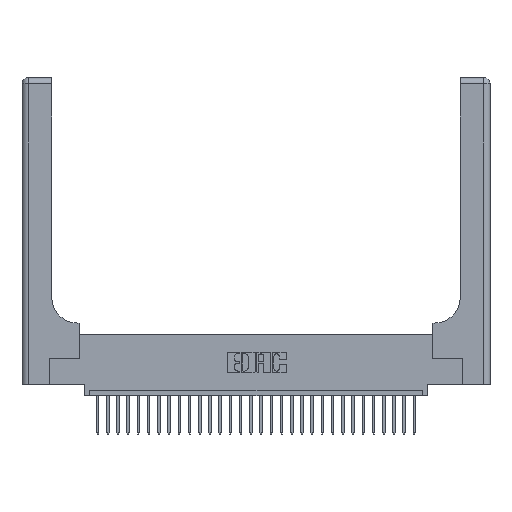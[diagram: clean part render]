
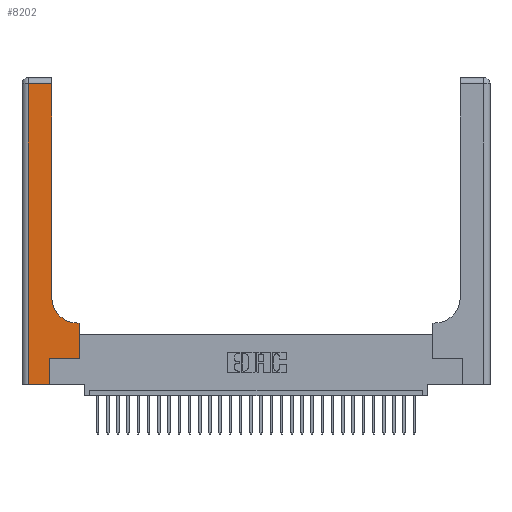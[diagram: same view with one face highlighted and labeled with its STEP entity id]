
A CAD part, top view. The second image highlights one B-rep face of the part: STEP entity #8202.
In plain terms, the highlighted planar face has unit normal (0, 0, 1).
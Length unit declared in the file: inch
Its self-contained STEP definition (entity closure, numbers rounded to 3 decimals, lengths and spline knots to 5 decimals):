
#45 = CARTESIAN_POINT ( 'NONE',  ( 0.06, 0., 0.37 ) ) ;
#70 = CARTESIAN_POINT ( 'NONE',  ( 0.2915, 3., 0.37 ) ) ;
#1363 = LINE ( 'NONE', #4420, #2109 ) ;
#1389 = CARTESIAN_POINT ( 'NONE',  ( 0., 3., 0.37 ) ) ;
#1496 = DIRECTION ( 'NONE',  ( -1., 0., 0. ) ) ;
#1990 = VERTEX_POINT ( 'NONE', #7342 ) ;
#2064 = LINE ( 'NONE', #16189, #18768 ) ;
#2109 = VECTOR ( 'NONE', #21030, 39.37008 ) ;
#2967 = CARTESIAN_POINT ( 'NONE',  ( 0.5415, 0.6, 0.37 ) ) ;
#3401 = CARTESIAN_POINT ( 'NONE',  ( 0.2915, 0.85, 0.37 ) ) ;
#3592 = LINE ( 'NONE', #70, #16576 ) ;
#4128 = DIRECTION ( 'NONE',  ( 0., 1., 0. ) ) ;
#4420 = CARTESIAN_POINT ( 'NONE',  ( 0., 0., 0.37 ) ) ;
#4796 = ORIENTED_EDGE ( 'NONE', *, *, #12431, .T. ) ;
#4954 = VECTOR ( 'NONE', #18918, 39.37008 ) ;
#4992 = ORIENTED_EDGE ( 'NONE', *, *, #6849, .T. ) ;
#5005 = EDGE_CURVE ( 'NONE', #25403, #25594, #29863, .T. ) ;
#5917 = CARTESIAN_POINT ( 'NONE',  ( 0.269, 0.25, 0.37 ) ) ;
#6511 = VERTEX_POINT ( 'NONE', #2967 ) ;
#6522 = EDGE_CURVE ( 'NONE', #28242, #1990, #15727, .T. ) ;
#6849 = EDGE_CURVE ( 'NONE', #29874, #8481, #12381, .T. ) ;
#7317 = CARTESIAN_POINT ( 'NONE',  ( 0.2915, 2.94, 0.37 ) ) ;
#7342 = CARTESIAN_POINT ( 'NONE',  ( 0.5585, 0.6, 0.37 ) ) ;
#8007 = DIRECTION ( 'NONE',  ( 1., 0., 0. ) ) ;
#8202 = ADVANCED_FACE ( 'NONE', ( #24514 ), #29800, .F. ) ;
#8350 = AXIS2_PLACEMENT_3D ( 'NONE', #26307, #9864, #19479 ) ;
#8481 = VERTEX_POINT ( 'NONE', #45 ) ;
#8844 = ORIENTED_EDGE ( 'NONE', *, *, #6522, .T. ) ;
#9443 = CARTESIAN_POINT ( 'NONE',  ( 0.269, 0., 0.37 ) ) ;
#9864 = DIRECTION ( 'NONE',  ( 0., 0., -1. ) ) ;
#10167 = CARTESIAN_POINT ( 'NONE',  ( 0.5585, 0.25, 0.37 ) ) ;
#11515 = CIRCLE ( 'NONE', #8350, 0.25 ) ;
#12280 = EDGE_CURVE ( 'NONE', #25594, #28242, #26995, .T. ) ;
#12381 = LINE ( 'NONE', #25745, #4954 ) ;
#12431 = EDGE_CURVE ( 'NONE', #26972, #29874, #18111, .T. ) ;
#12873 = EDGE_CURVE ( 'NONE', #14348, #26972, #3592, .T. ) ;
#13849 = CARTESIAN_POINT ( 'NONE',  ( 0.269, 0., 0.37 ) ) ;
#14348 = VERTEX_POINT ( 'NONE', #3401 ) ;
#15017 = ORIENTED_EDGE ( 'NONE', *, *, #17464, .T. ) ;
#15727 = LINE ( 'NONE', #10167, #21284 ) ;
#16189 = CARTESIAN_POINT ( 'NONE',  ( 0.2915, 0.6, 0.37 ) ) ;
#16576 = VECTOR ( 'NONE', #4128, 39.37008 ) ;
#17464 = EDGE_CURVE ( 'NONE', #1990, #6511, #2064, .T. ) ;
#18025 = DIRECTION ( 'NONE',  ( 0., 0., -1. ) ) ;
#18111 = LINE ( 'NONE', #29743, #28426 ) ;
#18121 = ORIENTED_EDGE ( 'NONE', *, *, #5005, .T. ) ;
#18755 = CARTESIAN_POINT ( 'NONE',  ( 0.5585, 0.25, 0.37 ) ) ;
#18768 = VECTOR ( 'NONE', #28164, 39.37008 ) ;
#18918 = DIRECTION ( 'NONE',  ( 0., -1., 0. ) ) ;
#19479 = DIRECTION ( 'NONE',  ( 1., 0., 0. ) ) ;
#19800 = ORIENTED_EDGE ( 'NONE', *, *, #28256, .T. ) ;
#20993 = CARTESIAN_POINT ( 'NONE',  ( 0.269, 0.25, 0.37 ) ) ;
#21030 = DIRECTION ( 'NONE',  ( 1., 0., 0. ) ) ;
#21284 = VECTOR ( 'NONE', #24417, 39.37008 ) ;
#21826 = ORIENTED_EDGE ( 'NONE', *, *, #12873, .T. ) ;
#23658 = ORIENTED_EDGE ( 'NONE', *, *, #12280, .T. ) ;
#24417 = DIRECTION ( 'NONE',  ( 0., 1., 0. ) ) ;
#24514 = FACE_OUTER_BOUND ( 'NONE', #28254, .T. ) ;
#24660 = VECTOR ( 'NONE', #28366, 39.37008 ) ;
#24974 = EDGE_CURVE ( 'NONE', #8481, #25403, #1363, .T. ) ;
#25198 = ORIENTED_EDGE ( 'NONE', *, *, #24974, .T. ) ;
#25403 = VERTEX_POINT ( 'NONE', #13849 ) ;
#25594 = VERTEX_POINT ( 'NONE', #20993 ) ;
#25745 = CARTESIAN_POINT ( 'NONE',  ( 0.06, 3., 0.37 ) ) ;
#26307 = CARTESIAN_POINT ( 'NONE',  ( 0.5415, 0.85, 0.37 ) ) ;
#26972 = VERTEX_POINT ( 'NONE', #7317 ) ;
#26995 = LINE ( 'NONE', #5917, #29970 ) ;
#27554 = DIRECTION ( 'NONE',  ( -1., 0., 0. ) ) ;
#28164 = DIRECTION ( 'NONE',  ( -1., 0., 0. ) ) ;
#28242 = VERTEX_POINT ( 'NONE', #18755 ) ;
#28254 = EDGE_LOOP ( 'NONE', ( #21826, #4796, #4992, #25198, #18121, #23658, #8844, #15017, #19800 ) ) ;
#28256 = EDGE_CURVE ( 'NONE', #6511, #14348, #11515, .T. ) ;
#28366 = DIRECTION ( 'NONE',  ( 0., 1., 0. ) ) ;
#28426 = VECTOR ( 'NONE', #27554, 39.37008 ) ;
#29267 = AXIS2_PLACEMENT_3D ( 'NONE', #1389, #18025, #1496 ) ;
#29743 = CARTESIAN_POINT ( 'NONE',  ( 0., 2.94, 0.37 ) ) ;
#29800 = PLANE ( 'NONE',  #29267 ) ;
#29863 = LINE ( 'NONE', #9443, #24660 ) ;
#29874 = VERTEX_POINT ( 'NONE', #30574 ) ;
#29970 = VECTOR ( 'NONE', #8007, 39.37008 ) ;
#30574 = CARTESIAN_POINT ( 'NONE',  ( 0.06, 2.94, 0.37 ) ) ;
